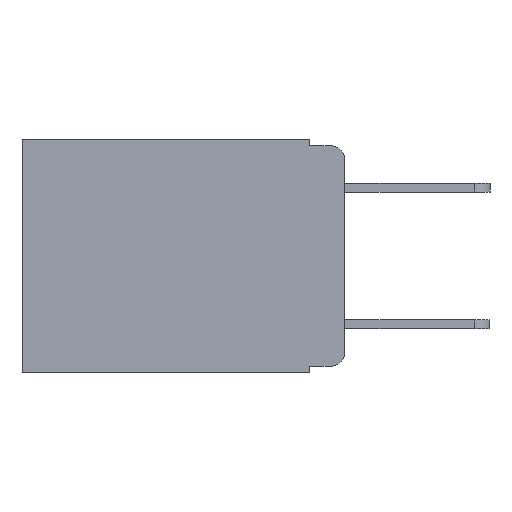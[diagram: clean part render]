
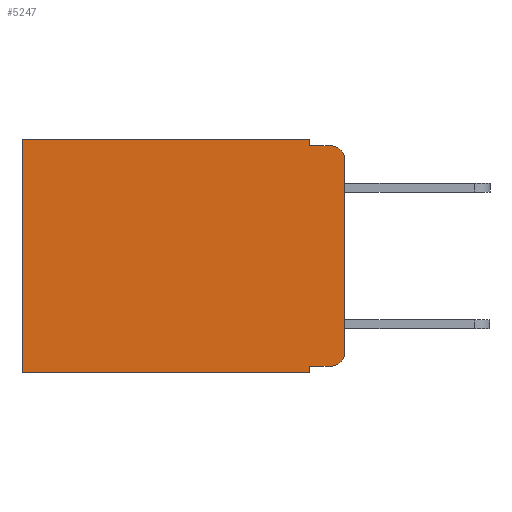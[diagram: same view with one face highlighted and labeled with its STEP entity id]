
A CAD part, left-side view. The second image highlights one B-rep face of the part: STEP entity #5247.
In plain terms, the highlighted planar face has unit normal (-1, 0, 0).
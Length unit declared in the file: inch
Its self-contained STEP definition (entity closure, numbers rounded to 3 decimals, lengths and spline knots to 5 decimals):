
#192 = DIRECTION ( 'NONE',  ( 0., 0., -1. ) ) ;
#354 = VERTEX_POINT ( 'NONE', #3644 ) ;
#377 = LINE ( 'NONE', #4832, #6566 ) ;
#395 = VERTEX_POINT ( 'NONE', #4888 ) ;
#439 = EDGE_CURVE ( 'NONE', #9591, #395, #8568, .T. ) ;
#480 = EDGE_CURVE ( 'NONE', #7502, #9591, #3984, .T. ) ;
#501 = VERTEX_POINT ( 'NONE', #4957 ) ;
#510 = LINE ( 'NONE', #7283, #6655 ) ;
#513 = CARTESIAN_POINT ( 'NONE',  ( 0.298, 0.051, -0.343 ) ) ;
#514 = EDGE_CURVE ( 'NONE', #7502, #6833, #9347, .T. ) ;
#516 = VERTEX_POINT ( 'NONE', #1413 ) ;
#605 = EDGE_CURVE ( 'NONE', #501, #6022, #510, .T. ) ;
#638 = DIRECTION ( 'NONE',  ( -1., 0., 0. ) ) ;
#866 = LINE ( 'NONE', #8042, #8485 ) ;
#903 = VECTOR ( 'NONE', #5885, 39.37008 ) ;
#1169 = EDGE_LOOP ( 'NONE', ( #2071, #2156, #2219, #2261, #2303, #2390, #2409, #2473, #2533, #2587 ) ) ;
#1359 = VECTOR ( 'NONE', #5533, 39.37008 ) ;
#1413 = CARTESIAN_POINT ( 'NONE',  ( 0.298, 0.051, -0.01 ) ) ;
#1418 = AXIS2_PLACEMENT_3D ( 'NONE', #8774, #9310, #7942 ) ;
#1445 = DIRECTION ( 'NONE',  ( 0., 0., -1. ) ) ;
#1641 = VECTOR ( 'NONE', #7075, 39.37008 ) ;
#1842 = LINE ( 'NONE', #5773, #5810 ) ;
#1935 = VERTEX_POINT ( 'NONE', #5699 ) ;
#2071 = ORIENTED_EDGE ( 'NONE', *, *, #8244, .F. ) ;
#2156 = ORIENTED_EDGE ( 'NONE', *, *, #7034, .T. ) ;
#2219 = ORIENTED_EDGE ( 'NONE', *, *, #6968, .F. ) ;
#2261 = ORIENTED_EDGE ( 'NONE', *, *, #4688, .F. ) ;
#2303 = ORIENTED_EDGE ( 'NONE', *, *, #5394, .T. ) ;
#2390 = ORIENTED_EDGE ( 'NONE', *, *, #605, .T. ) ;
#2409 = ORIENTED_EDGE ( 'NONE', *, *, #9638, .F. ) ;
#2473 = ORIENTED_EDGE ( 'NONE', *, *, #514, .F. ) ;
#2533 = ORIENTED_EDGE ( 'NONE', *, *, #480, .T. ) ;
#2587 = ORIENTED_EDGE ( 'NONE', *, *, #439, .T. ) ;
#2888 = CARTESIAN_POINT ( 'NONE',  ( 0.298, 0.051, 0. ) ) ;
#3037 = VECTOR ( 'NONE', #4134, 39.37008 ) ;
#3169 = AXIS2_PLACEMENT_3D ( 'NONE', #9687, #638, #192 ) ;
#3406 = DIRECTION ( 'NONE',  ( 0., 1., 0. ) ) ;
#3494 = VERTEX_POINT ( 'NONE', #3514 ) ;
#3514 = CARTESIAN_POINT ( 'NONE',  ( 0.298, 0., -0.03 ) ) ;
#3644 = CARTESIAN_POINT ( 'NONE',  ( 0.298, 0.051, 0. ) ) ;
#3984 = LINE ( 'NONE', #8915, #1641 ) ;
#4134 = DIRECTION ( 'NONE',  ( 0., 0., -1. ) ) ;
#4661 = FACE_OUTER_BOUND ( 'NONE', #1169, .T. ) ;
#4688 = EDGE_CURVE ( 'NONE', #354, #516, #8734, .T. ) ;
#4731 = CARTESIAN_POINT ( 'NONE',  ( 0.298, 0.051, -0.333 ) ) ;
#4832 = CARTESIAN_POINT ( 'NONE',  ( 0.298, 0., -0.343 ) ) ;
#4888 = CARTESIAN_POINT ( 'NONE',  ( 0.298, 0., -0.313 ) ) ;
#4957 = CARTESIAN_POINT ( 'NONE',  ( 0.298, 0.473, 0. ) ) ;
#5247 = ADVANCED_FACE ( 'NONE', ( #4661 ), #9147, .F. ) ;
#5257 = CIRCLE ( 'NONE', #6070, 0.02 ) ;
#5394 = EDGE_CURVE ( 'NONE', #354, #501, #866, .T. ) ;
#5533 = DIRECTION ( 'NONE',  ( 0., 0., -1. ) ) ;
#5699 = CARTESIAN_POINT ( 'NONE',  ( 0.298, 0.02, -0.01 ) ) ;
#5773 = CARTESIAN_POINT ( 'NONE',  ( 0.298, 0., 0. ) ) ;
#5810 = VECTOR ( 'NONE', #6495, 39.37008 ) ;
#5885 = DIRECTION ( 'NONE',  ( 0., -1., 0. ) ) ;
#6022 = VERTEX_POINT ( 'NONE', #7647 ) ;
#6070 = AXIS2_PLACEMENT_3D ( 'NONE', #6834, #8369, #8287 ) ;
#6495 = DIRECTION ( 'NONE',  ( 0., 0., -1. ) ) ;
#6566 = VECTOR ( 'NONE', #3406, 39.37008 ) ;
#6655 = VECTOR ( 'NONE', #1445, 39.37008 ) ;
#6833 = VERTEX_POINT ( 'NONE', #513 ) ;
#6834 = CARTESIAN_POINT ( 'NONE',  ( 0.298, 0.02, -0.03 ) ) ;
#6968 = EDGE_CURVE ( 'NONE', #516, #1935, #9639, .T. ) ;
#7034 = EDGE_CURVE ( 'NONE', #3494, #1935, #5257, .T. ) ;
#7075 = DIRECTION ( 'NONE',  ( 0., -1., 0. ) ) ;
#7283 = CARTESIAN_POINT ( 'NONE',  ( 0.298, 0.473, 0. ) ) ;
#7502 = VERTEX_POINT ( 'NONE', #4731 ) ;
#7647 = CARTESIAN_POINT ( 'NONE',  ( 0.298, 0.473, -0.343 ) ) ;
#7942 = DIRECTION ( 'NONE',  ( 0., 0., -1. ) ) ;
#8009 = DIRECTION ( 'NONE',  ( 0., 1., 0. ) ) ;
#8042 = CARTESIAN_POINT ( 'NONE',  ( 0.298, 0., 0. ) ) ;
#8244 = EDGE_CURVE ( 'NONE', #3494, #395, #1842, .T. ) ;
#8287 = DIRECTION ( 'NONE',  ( 0., 0., -1. ) ) ;
#8369 = DIRECTION ( 'NONE',  ( -1., 0., 0. ) ) ;
#8485 = VECTOR ( 'NONE', #8009, 39.37008 ) ;
#8568 = CIRCLE ( 'NONE', #3169, 0.02 ) ;
#8734 = LINE ( 'NONE', #2888, #3037 ) ;
#8774 = CARTESIAN_POINT ( 'NONE',  ( 0.298, 0., 0. ) ) ;
#8915 = CARTESIAN_POINT ( 'NONE',  ( 0.298, 0.051, -0.333 ) ) ;
#9001 = CARTESIAN_POINT ( 'NONE',  ( 0.298, 0.051, -0.01 ) ) ;
#9147 = PLANE ( 'NONE',  #1418 ) ;
#9310 = DIRECTION ( 'NONE',  ( 1., 0., 0. ) ) ;
#9347 = LINE ( 'NONE', #9442, #1359 ) ;
#9442 = CARTESIAN_POINT ( 'NONE',  ( 0.298, 0.051, 0. ) ) ;
#9591 = VERTEX_POINT ( 'NONE', #9658 ) ;
#9638 = EDGE_CURVE ( 'NONE', #6833, #6022, #377, .T. ) ;
#9639 = LINE ( 'NONE', #9001, #903 ) ;
#9658 = CARTESIAN_POINT ( 'NONE',  ( 0.298, 0.02, -0.333 ) ) ;
#9687 = CARTESIAN_POINT ( 'NONE',  ( 0.298, 0.02, -0.313 ) ) ;
